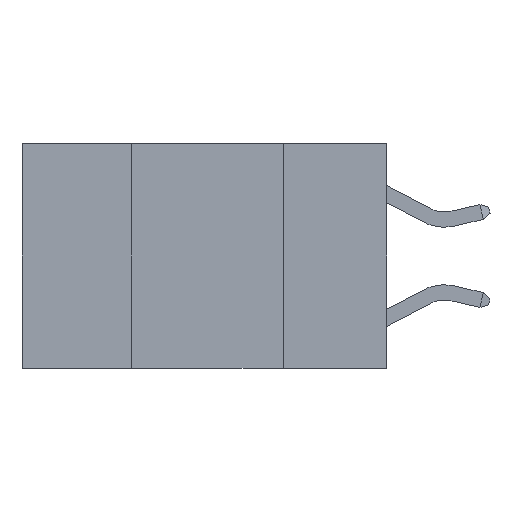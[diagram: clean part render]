
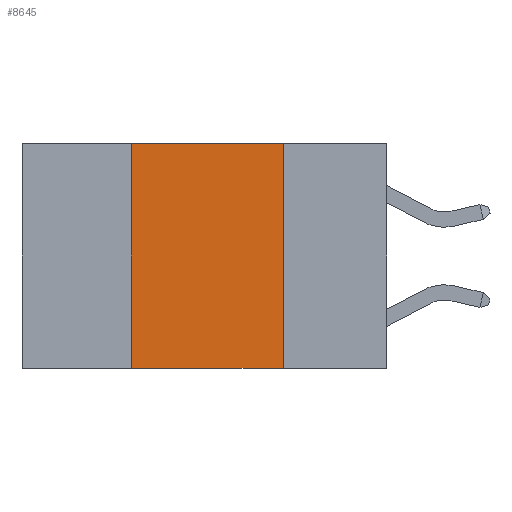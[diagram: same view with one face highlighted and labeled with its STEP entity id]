
A CAD part, left-side view. The second image highlights one B-rep face of the part: STEP entity #8645.
In plain terms, the highlighted planar face has unit normal (-1, 0, 0).
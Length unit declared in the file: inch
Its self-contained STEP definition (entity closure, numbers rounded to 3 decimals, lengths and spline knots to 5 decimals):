
#255 = FACE_OUTER_BOUND ( 'NONE', #1119, .T. ) ;
#266 = DIRECTION ( 'NONE',  ( 0., 0., 1. ) ) ;
#984 = LINE ( 'NONE', #8209, #5314 ) ;
#1034 = DIRECTION ( 'NONE',  ( 0., -1., 0. ) ) ;
#1119 = EDGE_LOOP ( 'NONE', ( #8719, #1907, #6371, #2994 ) ) ;
#1153 = CARTESIAN_POINT ( 'NONE',  ( 0., 0.17, -0.37 ) ) ;
#1410 = CARTESIAN_POINT ( 'NONE',  ( 0., 0.42, 0. ) ) ;
#1664 = EDGE_CURVE ( 'NONE', #1732, #3140, #1925, .T. ) ;
#1732 = VERTEX_POINT ( 'NONE', #8986 ) ;
#1907 = ORIENTED_EDGE ( 'NONE', *, *, #7822, .F. ) ;
#1925 = LINE ( 'NONE', #7226, #2800 ) ;
#2571 = VERTEX_POINT ( 'NONE', #1153 ) ;
#2631 = DIRECTION ( 'NONE',  ( 1., 0., 0. ) ) ;
#2685 = CARTESIAN_POINT ( 'NONE',  ( 0., 0.6, 0. ) ) ;
#2800 = VECTOR ( 'NONE', #266, 39.37008 ) ;
#2994 = ORIENTED_EDGE ( 'NONE', *, *, #6534, .T. ) ;
#3055 = AXIS2_PLACEMENT_3D ( 'NONE', #2685, #2631, #7945 ) ;
#3140 = VERTEX_POINT ( 'NONE', #1410 ) ;
#3185 = DIRECTION ( 'NONE',  ( 0., 0., -1. ) ) ;
#3359 = PLANE ( 'NONE',  #3055 ) ;
#3396 = CARTESIAN_POINT ( 'NONE',  ( 0., 0.6, 0. ) ) ;
#4164 = VERTEX_POINT ( 'NONE', #5489 ) ;
#5314 = VECTOR ( 'NONE', #5600, 39.37008 ) ;
#5489 = CARTESIAN_POINT ( 'NONE',  ( 0., 0.17, 0. ) ) ;
#5600 = DIRECTION ( 'NONE',  ( 0., -1., 0. ) ) ;
#6132 = VECTOR ( 'NONE', #1034, 39.37008 ) ;
#6371 = ORIENTED_EDGE ( 'NONE', *, *, #1664, .F. ) ;
#6534 = EDGE_CURVE ( 'NONE', #1732, #2571, #984, .T. ) ;
#6948 = LINE ( 'NONE', #9339, #9862 ) ;
#7226 = CARTESIAN_POINT ( 'NONE',  ( 0., 0.42, 0. ) ) ;
#7822 = EDGE_CURVE ( 'NONE', #3140, #4164, #8687, .T. ) ;
#7945 = DIRECTION ( 'NONE',  ( 0., 0., -1. ) ) ;
#8187 = EDGE_CURVE ( 'NONE', #4164, #2571, #6948, .T. ) ;
#8209 = CARTESIAN_POINT ( 'NONE',  ( 0., 0.6, -0.37 ) ) ;
#8645 = ADVANCED_FACE ( 'NONE', ( #255 ), #3359, .F. ) ;
#8687 = LINE ( 'NONE', #3396, #6132 ) ;
#8719 = ORIENTED_EDGE ( 'NONE', *, *, #8187, .F. ) ;
#8986 = CARTESIAN_POINT ( 'NONE',  ( 0., 0.42, -0.37 ) ) ;
#9339 = CARTESIAN_POINT ( 'NONE',  ( 0., 0.17, 0. ) ) ;
#9862 = VECTOR ( 'NONE', #3185, 39.37008 ) ;
